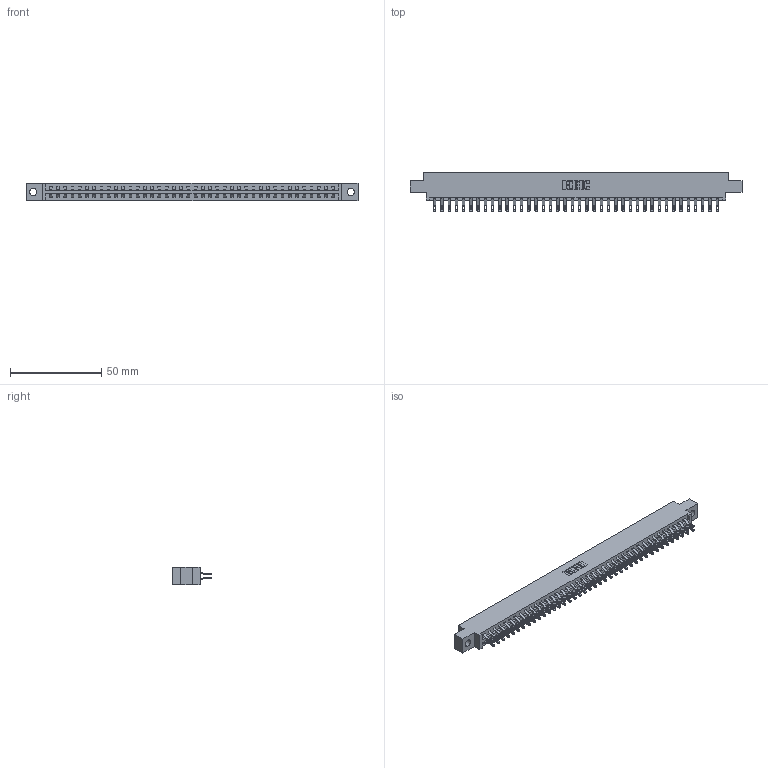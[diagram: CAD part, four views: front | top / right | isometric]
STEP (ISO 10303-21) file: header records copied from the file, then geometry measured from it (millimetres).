
FILE_DESCRIPTION (( 'STEP AP203' ), '1' );
FILE_NAME ('337-080-555-804.STEP', '2018-08-12T18:37:24', ( '' ), ( '' ), 'SwSTEP 2.0', 'SolidWorks 2016', '' );
FILE_SCHEMA (( 'CONFIG_CONTROL_DESIGN' ));
Length unit declared in the file: inch
Products named in the file (3): 337 Part_0.170 Offset - 0.156 Dia-TH; 345-292-001_555 Tail; 337-080-555-804
Assembly tree (81 placements, depth 2):
  337-080-555-804
    337 Part_0.170 Offset - 0.156 Dia-TH
    345-292-001_555 Tail  x80
Bounding box: 181.51 x 21.47 x 9.4 mm (x, y, z)
Volume: 19128.9 mm3; surface area: 22385.5 mm2
Topology: 81 solids, 81 shells, 4918 faces, 15443 edges, 10294 vertices
Faces by surface type: plane 2954, cylinder 1964
Entity records: 31733 total; most frequent: CARTESIAN_POINT 5384, ORIENTED_EDGE 5290, DIRECTION 4553, EDGE_CURVE 2645, LINE 2497, VECTOR 2497, VERTEX_POINT 1762, AXIS2_PLACEMENT_3D 1028
